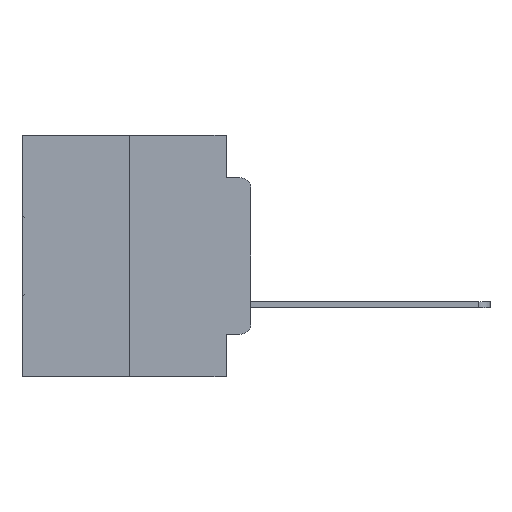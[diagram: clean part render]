
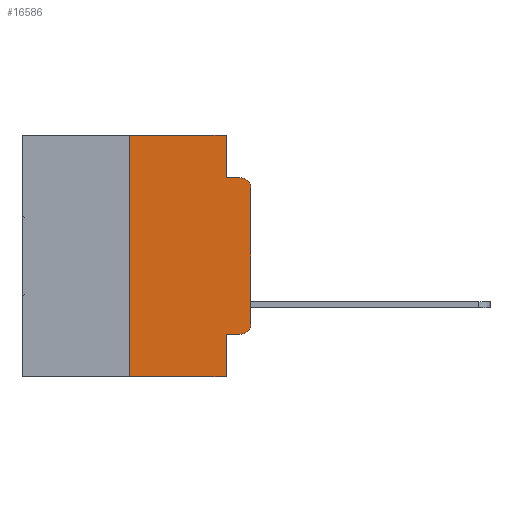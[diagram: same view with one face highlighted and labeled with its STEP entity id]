
A CAD part, left-side view. The second image highlights one B-rep face of the part: STEP entity #16586.
In plain terms, the highlighted planar face has unit normal (-1, 0, 0).
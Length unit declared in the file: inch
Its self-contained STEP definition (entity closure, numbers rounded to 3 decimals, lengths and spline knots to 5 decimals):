
#341 = AXIS2_PLACEMENT_3D ( 'NONE', #962, #18996, #3619 ) ;
#561 = FACE_OUTER_BOUND ( 'NONE', #14590, .T. ) ;
#962 = CARTESIAN_POINT ( 'NONE',  ( 0., 0.02, -0.1085 ) ) ;
#1006 = CARTESIAN_POINT ( 'NONE',  ( 0., 0.25, -0.5 ) ) ;
#1055 = ORIENTED_EDGE ( 'NONE', *, *, #13274, .T. ) ;
#1472 = ORIENTED_EDGE ( 'NONE', *, *, #9486, .T. ) ;
#1642 = LINE ( 'NONE', #19068, #27721 ) ;
#2318 = CARTESIAN_POINT ( 'NONE',  ( 0., 0.051, -0.4115 ) ) ;
#2512 = EDGE_CURVE ( 'NONE', #25723, #8986, #28311, .T. ) ;
#3166 = EDGE_CURVE ( 'NONE', #3446, #19254, #15562, .T. ) ;
#3446 = VERTEX_POINT ( 'NONE', #2318 ) ;
#3619 = DIRECTION ( 'NONE',  ( 0., 0., -1. ) ) ;
#3657 = VECTOR ( 'NONE', #8572, 39.37008 ) ;
#3794 = DIRECTION ( 'NONE',  ( 0., 0., -1. ) ) ;
#4146 = VECTOR ( 'NONE', #29865, 39.37008 ) ;
#4154 = LINE ( 'NONE', #18616, #30006 ) ;
#4744 = CARTESIAN_POINT ( 'NONE',  ( 0., 0., -0.1085 ) ) ;
#4865 = EDGE_CURVE ( 'NONE', #6862, #31383, #4154, .T. ) ;
#5563 = ORIENTED_EDGE ( 'NONE', *, *, #6238, .F. ) ;
#6029 = CARTESIAN_POINT ( 'NONE',  ( 0., 0., -0.3915 ) ) ;
#6238 = EDGE_CURVE ( 'NONE', #31383, #31794, #30270, .T. ) ;
#6576 = CARTESIAN_POINT ( 'NONE',  ( 0., 0.051, -0.5 ) ) ;
#6862 = VERTEX_POINT ( 'NONE', #1006 ) ;
#7173 = CARTESIAN_POINT ( 'NONE',  ( 0., 0., 0. ) ) ;
#8572 = DIRECTION ( 'NONE',  ( 0., -1., 0. ) ) ;
#8678 = CARTESIAN_POINT ( 'NONE',  ( 0., 0.051, 0. ) ) ;
#8929 = CARTESIAN_POINT ( 'NONE',  ( 0., 0.02, -0.0885 ) ) ;
#8986 = VERTEX_POINT ( 'NONE', #8929 ) ;
#9108 = CARTESIAN_POINT ( 'NONE',  ( 0., 0.02, -0.3915 ) ) ;
#9486 = EDGE_CURVE ( 'NONE', #30503, #25723, #19070, .T. ) ;
#10026 = ORIENTED_EDGE ( 'NONE', *, *, #13477, .F. ) ;
#10109 = EDGE_CURVE ( 'NONE', #31794, #29136, #19421, .T. ) ;
#10417 = DIRECTION ( 'NONE',  ( 1., 0., 0. ) ) ;
#10435 = ORIENTED_EDGE ( 'NONE', *, *, #30608, .T. ) ;
#11474 = DIRECTION ( 'NONE',  ( 0., -1., 0. ) ) ;
#11646 = DIRECTION ( 'NONE',  ( 0., 0., -1. ) ) ;
#11664 = AXIS2_PLACEMENT_3D ( 'NONE', #9108, #26619, #11646 ) ;
#11820 = CARTESIAN_POINT ( 'NONE',  ( 0., 0.02, -0.4115 ) ) ;
#12011 = CARTESIAN_POINT ( 'NONE',  ( 0., 0.051, -0.0885 ) ) ;
#12255 = VECTOR ( 'NONE', #29602, 39.37008 ) ;
#12973 = CARTESIAN_POINT ( 'NONE',  ( 0., 0.051, -0.4115 ) ) ;
#13274 = EDGE_CURVE ( 'NONE', #6862, #19254, #1642, .T. ) ;
#13477 = EDGE_CURVE ( 'NONE', #29136, #8986, #29563, .T. ) ;
#13674 = CARTESIAN_POINT ( 'NONE',  ( 0., 0.473, 0. ) ) ;
#14590 = EDGE_LOOP ( 'NONE', ( #1472, #21930, #10026, #29784, #5563, #25710, #1055, #14795, #27949, #10435 ) ) ;
#14795 = ORIENTED_EDGE ( 'NONE', *, *, #3166, .F. ) ;
#15058 = CARTESIAN_POINT ( 'NONE',  ( 0., 0.051, 0. ) ) ;
#15468 = DIRECTION ( 'NONE',  ( 0., -1., 0. ) ) ;
#15562 = LINE ( 'NONE', #26553, #21517 ) ;
#16548 = VECTOR ( 'NONE', #24565, 39.37008 ) ;
#16586 = ADVANCED_FACE ( 'NONE', ( #561 ), #32507, .F. ) ;
#16877 = VERTEX_POINT ( 'NONE', #11820 ) ;
#18616 = CARTESIAN_POINT ( 'NONE',  ( 0., 0.25, 0. ) ) ;
#18996 = DIRECTION ( 'NONE',  ( -1., 0., 0. ) ) ;
#19068 = CARTESIAN_POINT ( 'NONE',  ( 0., 0.473, -0.5 ) ) ;
#19070 = LINE ( 'NONE', #7173, #12255 ) ;
#19254 = VERTEX_POINT ( 'NONE', #6576 ) ;
#19421 = LINE ( 'NONE', #15058, #4146 ) ;
#21517 = VECTOR ( 'NONE', #3794, 39.37008 ) ;
#21930 = ORIENTED_EDGE ( 'NONE', *, *, #2512, .T. ) ;
#22637 = CIRCLE ( 'NONE', #11664, 0.02 ) ;
#24462 = LINE ( 'NONE', #12973, #29283 ) ;
#24565 = DIRECTION ( 'NONE',  ( 0., -1., 0. ) ) ;
#25447 = CARTESIAN_POINT ( 'NONE',  ( 0., 0.473, 0. ) ) ;
#25710 = ORIENTED_EDGE ( 'NONE', *, *, #4865, .F. ) ;
#25723 = VERTEX_POINT ( 'NONE', #4744 ) ;
#26553 = CARTESIAN_POINT ( 'NONE',  ( 0., 0.051, 0. ) ) ;
#26619 = DIRECTION ( 'NONE',  ( -1., 0., 0. ) ) ;
#27486 = AXIS2_PLACEMENT_3D ( 'NONE', #25447, #10417, #27827 ) ;
#27721 = VECTOR ( 'NONE', #11474, 39.37008 ) ;
#27827 = DIRECTION ( 'NONE',  ( 0., 0., -1. ) ) ;
#27949 = ORIENTED_EDGE ( 'NONE', *, *, #32221, .T. ) ;
#28281 = CARTESIAN_POINT ( 'NONE',  ( 0., 0.051, -0.0885 ) ) ;
#28311 = CIRCLE ( 'NONE', #341, 0.02 ) ;
#29136 = VERTEX_POINT ( 'NONE', #28281 ) ;
#29283 = VECTOR ( 'NONE', #15468, 39.37008 ) ;
#29563 = LINE ( 'NONE', #12011, #16548 ) ;
#29567 = CARTESIAN_POINT ( 'NONE',  ( 0., 0.25, 0. ) ) ;
#29602 = DIRECTION ( 'NONE',  ( 0., 0., 1. ) ) ;
#29784 = ORIENTED_EDGE ( 'NONE', *, *, #10109, .F. ) ;
#29865 = DIRECTION ( 'NONE',  ( 0., 0., -1. ) ) ;
#30006 = VECTOR ( 'NONE', #30775, 39.37008 ) ;
#30270 = LINE ( 'NONE', #13674, #3657 ) ;
#30503 = VERTEX_POINT ( 'NONE', #6029 ) ;
#30608 = EDGE_CURVE ( 'NONE', #16877, #30503, #22637, .T. ) ;
#30775 = DIRECTION ( 'NONE',  ( 0., 0., 1. ) ) ;
#31383 = VERTEX_POINT ( 'NONE', #29567 ) ;
#31794 = VERTEX_POINT ( 'NONE', #8678 ) ;
#32221 = EDGE_CURVE ( 'NONE', #3446, #16877, #24462, .T. ) ;
#32507 = PLANE ( 'NONE',  #27486 ) ;
